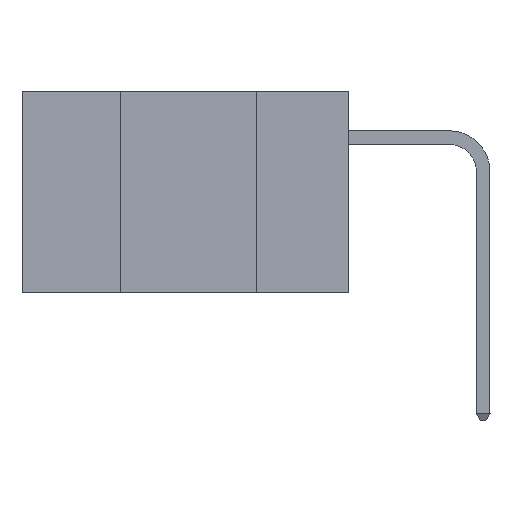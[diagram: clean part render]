
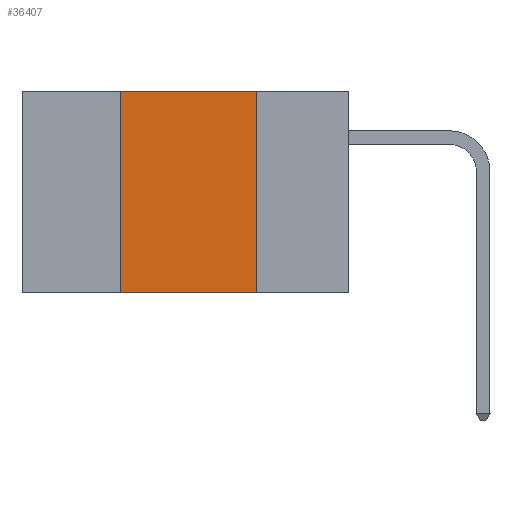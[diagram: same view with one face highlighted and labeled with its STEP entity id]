
A CAD part, left-side view. The second image highlights one B-rep face of the part: STEP entity #36407.
In plain terms, the highlighted planar face has unit normal (-1, 0, 0).
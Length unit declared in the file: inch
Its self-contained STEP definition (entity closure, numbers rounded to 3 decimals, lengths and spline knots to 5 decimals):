
#333 = PLANE ( 'NONE',  #24491 ) ;
#2055 = CARTESIAN_POINT ( 'NONE',  ( 0., 0.17, 0. ) ) ;
#2084 = LINE ( 'NONE', #29769, #18630 ) ;
#4653 = EDGE_CURVE ( 'NONE', #16213, #32101, #2084, .T. ) ;
#4727 = CARTESIAN_POINT ( 'NONE',  ( 0., 0.6, 0. ) ) ;
#6740 = DIRECTION ( 'NONE',  ( 1., 0., 0. ) ) ;
#8111 = VERTEX_POINT ( 'NONE', #2055 ) ;
#8480 = LINE ( 'NONE', #39577, #11624 ) ;
#9355 = ORIENTED_EDGE ( 'NONE', *, *, #35421, .T. ) ;
#9574 = FACE_OUTER_BOUND ( 'NONE', #33659, .T. ) ;
#11156 = DIRECTION ( 'NONE',  ( 0., -1., 0. ) ) ;
#11624 = VECTOR ( 'NONE', #38985, 39.37008 ) ;
#15037 = EDGE_CURVE ( 'NONE', #8111, #28317, #28331, .T. ) ;
#15517 = DIRECTION ( 'NONE',  ( 0., 0., -1. ) ) ;
#16213 = VERTEX_POINT ( 'NONE', #36182 ) ;
#18630 = VECTOR ( 'NONE', #26566, 39.37008 ) ;
#21225 = CARTESIAN_POINT ( 'NONE',  ( 0., 0.6, 0. ) ) ;
#21306 = CARTESIAN_POINT ( 'NONE',  ( 0., 0.42, 0. ) ) ;
#21470 = EDGE_CURVE ( 'NONE', #32101, #8111, #31624, .T. ) ;
#24491 = AXIS2_PLACEMENT_3D ( 'NONE', #21225, #6740, #24623 ) ;
#24623 = DIRECTION ( 'NONE',  ( 0., 0., -1. ) ) ;
#25097 = ORIENTED_EDGE ( 'NONE', *, *, #21470, .F. ) ;
#25131 = CARTESIAN_POINT ( 'NONE',  ( 0., 0.17, 0. ) ) ;
#25520 = ORIENTED_EDGE ( 'NONE', *, *, #15037, .F. ) ;
#26566 = DIRECTION ( 'NONE',  ( 0., 0., 1. ) ) ;
#27375 = VECTOR ( 'NONE', #15517, 39.37008 ) ;
#28317 = VERTEX_POINT ( 'NONE', #35433 ) ;
#28331 = LINE ( 'NONE', #25131, #27375 ) ;
#29605 = VECTOR ( 'NONE', #11156, 39.37008 ) ;
#29769 = CARTESIAN_POINT ( 'NONE',  ( 0., 0.42, 0. ) ) ;
#31624 = LINE ( 'NONE', #4727, #29605 ) ;
#32101 = VERTEX_POINT ( 'NONE', #21306 ) ;
#33659 = EDGE_LOOP ( 'NONE', ( #25520, #25097, #35741, #9355 ) ) ;
#35421 = EDGE_CURVE ( 'NONE', #16213, #28317, #8480, .T. ) ;
#35433 = CARTESIAN_POINT ( 'NONE',  ( 0., 0.17, -0.37 ) ) ;
#35741 = ORIENTED_EDGE ( 'NONE', *, *, #4653, .F. ) ;
#36182 = CARTESIAN_POINT ( 'NONE',  ( 0., 0.42, -0.37 ) ) ;
#36407 = ADVANCED_FACE ( 'NONE', ( #9574 ), #333, .F. ) ;
#38985 = DIRECTION ( 'NONE',  ( 0., -1., 0. ) ) ;
#39577 = CARTESIAN_POINT ( 'NONE',  ( 0., 0.6, -0.37 ) ) ;
